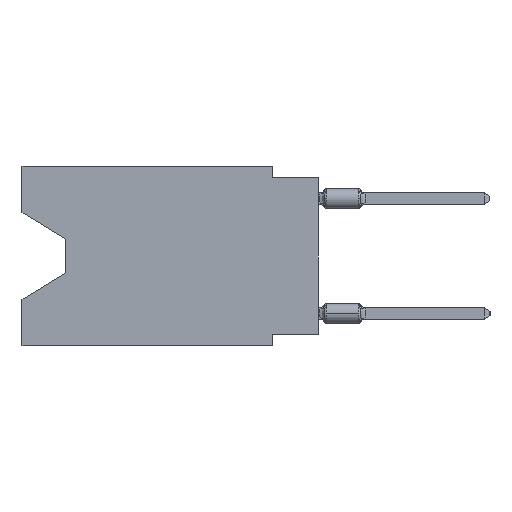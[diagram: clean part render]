
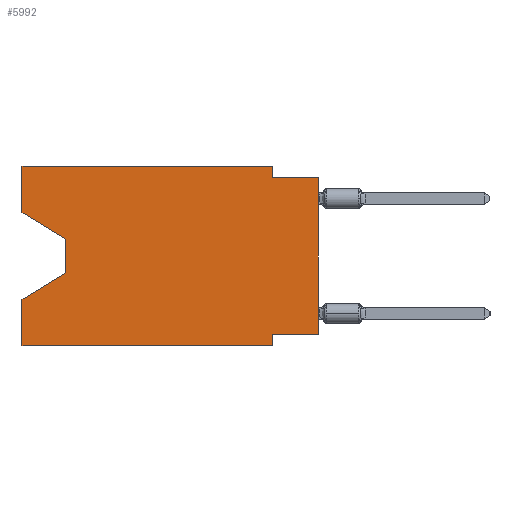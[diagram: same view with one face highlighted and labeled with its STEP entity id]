
A CAD part, left-side view. The second image highlights one B-rep face of the part: STEP entity #5992.
In plain terms, the highlighted planar face has unit normal (-1, 0, 0).
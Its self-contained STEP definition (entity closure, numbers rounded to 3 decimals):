
#150 = ORIENTED_EDGE ( 'NONE', *, *, #6593, .T. ) ;
#1283 = CARTESIAN_POINT ( 'NONE',  ( 0., 13.97, -5.893 ) ) ;
#1344 = DIRECTION ( 'NONE',  ( 0., 0., -1. ) ) ;
#1553 = ORIENTED_EDGE ( 'NONE', *, *, #16556, .F. ) ;
#1892 = CARTESIAN_POINT ( 'NONE',  ( 0., 16.383, 0. ) ) ;
#2563 = CARTESIAN_POINT ( 'NONE',  ( 0., 16.383, -7.36 ) ) ;
#2872 = VERTEX_POINT ( 'NONE', #1283 ) ;
#3258 = ORIENTED_EDGE ( 'NONE', *, *, #31104, .F. ) ;
#3999 = CARTESIAN_POINT ( 'NONE',  ( 0., 2.54, -9.906 ) ) ;
#5804 = VECTOR ( 'NONE', #35536, 1000. ) ;
#5992 = ADVANCED_FACE ( 'NONE', ( #29721 ), #48853, .F. ) ;
#6053 = LINE ( 'NONE', #21944, #34821 ) ;
#6507 = LINE ( 'NONE', #7441, #29597 ) ;
#6523 = DIRECTION ( 'NONE',  ( 0., -1., 0. ) ) ;
#6593 = EDGE_CURVE ( 'NONE', #26208, #22087, #25526, .T. ) ;
#7441 = CARTESIAN_POINT ( 'NONE',  ( 0., 16.383, -2.546 ) ) ;
#7518 = DIRECTION ( 'NONE',  ( 0., -1., 0. ) ) ;
#8662 = CARTESIAN_POINT ( 'NONE',  ( 0., 13.97, -4.013 ) ) ;
#8695 = ORIENTED_EDGE ( 'NONE', *, *, #19880, .F. ) ;
#9721 = ORIENTED_EDGE ( 'NONE', *, *, #48582, .F. ) ;
#9817 = CARTESIAN_POINT ( 'NONE',  ( 0., 16.383, 0. ) ) ;
#11232 = LINE ( 'NONE', #49509, #30332 ) ;
#11853 = CARTESIAN_POINT ( 'NONE',  ( 0., 0., -0.635 ) ) ;
#13511 = VECTOR ( 'NONE', #33673, 1000. ) ;
#13646 = CARTESIAN_POINT ( 'NONE',  ( 0., 16.383, 0. ) ) ;
#14518 = ORIENTED_EDGE ( 'NONE', *, *, #15498, .T. ) ;
#14628 = VERTEX_POINT ( 'NONE', #30353 ) ;
#14825 = LINE ( 'NONE', #9817, #13511 ) ;
#15498 = EDGE_CURVE ( 'NONE', #2872, #53457, #44955, .T. ) ;
#16187 = VECTOR ( 'NONE', #1344, 1000. ) ;
#16556 = EDGE_CURVE ( 'NONE', #25181, #23270, #51306, .T. ) ;
#17785 = CARTESIAN_POINT ( 'NONE',  ( 0., 13.97, -4.013 ) ) ;
#17944 = VECTOR ( 'NONE', #23592, 1000. ) ;
#19182 = VECTOR ( 'NONE', #34842, 1000. ) ;
#19880 = EDGE_CURVE ( 'NONE', #39158, #20903, #53757, .T. ) ;
#20000 = CARTESIAN_POINT ( 'NONE',  ( 0., 2.54, -0.635 ) ) ;
#20794 = DIRECTION ( 'NONE',  ( 0., 0., 1. ) ) ;
#20903 = VERTEX_POINT ( 'NONE', #3999 ) ;
#21944 = CARTESIAN_POINT ( 'NONE',  ( 0., 0., -0.635 ) ) ;
#22087 = VERTEX_POINT ( 'NONE', #11853 ) ;
#23054 = DIRECTION ( 'NONE',  ( 1., 0., 0. ) ) ;
#23270 = VERTEX_POINT ( 'NONE', #30987 ) ;
#23539 = ORIENTED_EDGE ( 'NONE', *, *, #26890, .T. ) ;
#23592 = DIRECTION ( 'NONE',  ( 0., 0., -1. ) ) ;
#23879 = EDGE_CURVE ( 'NONE', #23270, #59431, #25746, .T. ) ;
#24189 = CARTESIAN_POINT ( 'NONE',  ( 0., 0., -9.271 ) ) ;
#24547 = CARTESIAN_POINT ( 'NONE',  ( 0., 2.54, -9.271 ) ) ;
#24937 = VECTOR ( 'NONE', #51613, 1000. ) ;
#25181 = VERTEX_POINT ( 'NONE', #55007 ) ;
#25526 = LINE ( 'NONE', #34620, #59377 ) ;
#25746 = LINE ( 'NONE', #1892, #19182 ) ;
#26208 = VERTEX_POINT ( 'NONE', #24189 ) ;
#26665 = EDGE_CURVE ( 'NONE', #25181, #46415, #6507, .T. ) ;
#26890 = EDGE_CURVE ( 'NONE', #46415, #2872, #61105, .T. ) ;
#27777 = CARTESIAN_POINT ( 'NONE',  ( 0., 16.383, 0. ) ) ;
#29123 = EDGE_LOOP ( 'NONE', ( #52179, #23539, #14518, #47059, #61016, #8695, #9721, #150, #3258, #45501, #48029, #1553 ) ) ;
#29597 = VECTOR ( 'NONE', #55146, 1000. ) ;
#29721 = FACE_OUTER_BOUND ( 'NONE', #29123, .T. ) ;
#30332 = VECTOR ( 'NONE', #6523, 1000. ) ;
#30353 = CARTESIAN_POINT ( 'NONE',  ( 0., 16.383, -9.906 ) ) ;
#30653 = DIRECTION ( 'NONE',  ( 0., 1., 0. ) ) ;
#30987 = CARTESIAN_POINT ( 'NONE',  ( 0., 16.383, 0. ) ) ;
#31104 = EDGE_CURVE ( 'NONE', #43964, #22087, #6053, .T. ) ;
#32662 = EDGE_CURVE ( 'NONE', #59431, #43964, #48065, .T. ) ;
#33673 = DIRECTION ( 'NONE',  ( 0., 0., 1. ) ) ;
#33934 = CARTESIAN_POINT ( 'NONE',  ( 0., 2.54, 0. ) ) ;
#34539 = CARTESIAN_POINT ( 'NONE',  ( 0., 2.54, 0. ) ) ;
#34620 = CARTESIAN_POINT ( 'NONE',  ( 0., 0., 0. ) ) ;
#34821 = VECTOR ( 'NONE', #7518, 1000. ) ;
#34842 = DIRECTION ( 'NONE',  ( 0., -1., 0. ) ) ;
#35058 = LINE ( 'NONE', #48884, #38536 ) ;
#35536 = DIRECTION ( 'NONE',  ( 0., 0.855, -0.519 ) ) ;
#38536 = VECTOR ( 'NONE', #30653, 1000. ) ;
#39158 = VERTEX_POINT ( 'NONE', #24547 ) ;
#40279 = AXIS2_PLACEMENT_3D ( 'NONE', #13646, #23054, #43129 ) ;
#40607 = VECTOR ( 'NONE', #56078, 1000. ) ;
#43129 = DIRECTION ( 'NONE',  ( 0., 0., -1. ) ) ;
#43964 = VERTEX_POINT ( 'NONE', #20000 ) ;
#44351 = CARTESIAN_POINT ( 'NONE',  ( 0., 2.54, -9.906 ) ) ;
#44955 = LINE ( 'NONE', #54069, #5804 ) ;
#45501 = ORIENTED_EDGE ( 'NONE', *, *, #32662, .F. ) ;
#46415 = VERTEX_POINT ( 'NONE', #8662 ) ;
#47059 = ORIENTED_EDGE ( 'NONE', *, *, #48103, .F. ) ;
#48029 = ORIENTED_EDGE ( 'NONE', *, *, #23879, .F. ) ;
#48065 = LINE ( 'NONE', #34539, #17944 ) ;
#48103 = EDGE_CURVE ( 'NONE', #14628, #53457, #14825, .T. ) ;
#48582 = EDGE_CURVE ( 'NONE', #26208, #39158, #35058, .T. ) ;
#48853 = PLANE ( 'NONE',  #40279 ) ;
#48884 = CARTESIAN_POINT ( 'NONE',  ( 0., 0., -9.271 ) ) ;
#49509 = CARTESIAN_POINT ( 'NONE',  ( 0., 16.383, -9.906 ) ) ;
#51306 = LINE ( 'NONE', #27777, #24937 ) ;
#51613 = DIRECTION ( 'NONE',  ( 0., 0., 1. ) ) ;
#52179 = ORIENTED_EDGE ( 'NONE', *, *, #26665, .T. ) ;
#53457 = VERTEX_POINT ( 'NONE', #2563 ) ;
#53757 = LINE ( 'NONE', #44351, #16187 ) ;
#54069 = CARTESIAN_POINT ( 'NONE',  ( 0., 13.97, -5.893 ) ) ;
#55007 = CARTESIAN_POINT ( 'NONE',  ( 0., 16.383, -2.546 ) ) ;
#55146 = DIRECTION ( 'NONE',  ( 0., -0.855, -0.519 ) ) ;
#56078 = DIRECTION ( 'NONE',  ( 0., 0., -1. ) ) ;
#58232 = EDGE_CURVE ( 'NONE', #14628, #20903, #11232, .T. ) ;
#59377 = VECTOR ( 'NONE', #20794, 1000. ) ;
#59431 = VERTEX_POINT ( 'NONE', #33934 ) ;
#61016 = ORIENTED_EDGE ( 'NONE', *, *, #58232, .T. ) ;
#61105 = LINE ( 'NONE', #17785, #40607 ) ;
